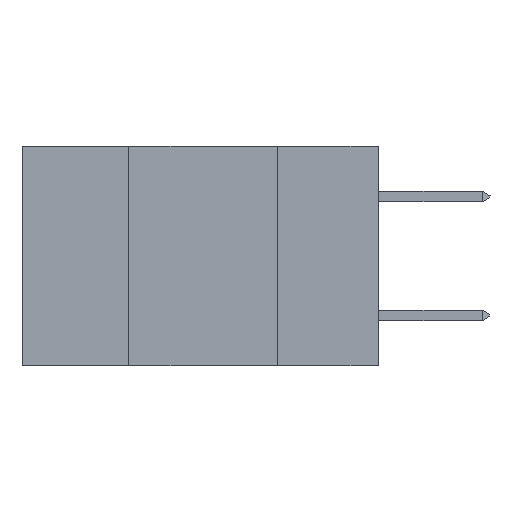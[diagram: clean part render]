
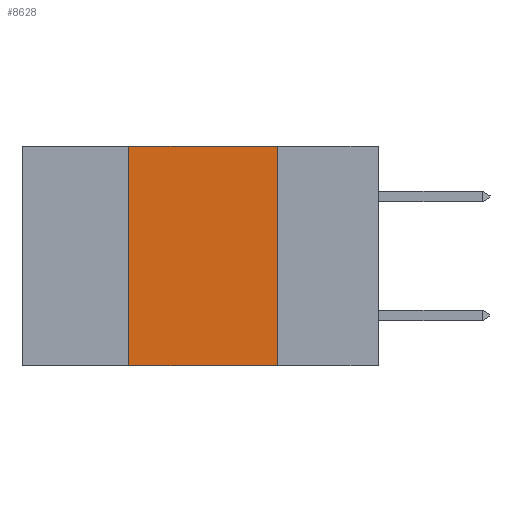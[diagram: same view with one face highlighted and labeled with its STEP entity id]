
A CAD part, left-side view. The second image highlights one B-rep face of the part: STEP entity #8628.
In plain terms, the highlighted planar face has unit normal (-1, 0, 0).
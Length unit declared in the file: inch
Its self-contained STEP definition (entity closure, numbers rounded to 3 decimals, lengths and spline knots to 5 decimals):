
#467 = CARTESIAN_POINT ( 'NONE',  ( 0., 0.6, 0. ) ) ;
#910 = CARTESIAN_POINT ( 'NONE',  ( 0., 0.17, -0.37 ) ) ;
#999 = ORIENTED_EDGE ( 'NONE', *, *, #2778, .F. ) ;
#1193 = CARTESIAN_POINT ( 'NONE',  ( 0., 0.17, -0.37 ) ) ;
#1244 = EDGE_CURVE ( 'NONE', #10765, #5327, #7498, .T. ) ;
#1844 = LINE ( 'NONE', #2875, #10966 ) ;
#1901 = ORIENTED_EDGE ( 'NONE', *, *, #1244, .T. ) ;
#2778 = EDGE_CURVE ( 'NONE', #9141, #6094, #1844, .T. ) ;
#2875 = CARTESIAN_POINT ( 'NONE',  ( 0., 0.6, 0. ) ) ;
#2904 = LINE ( 'NONE', #9290, #5956 ) ;
#3228 = VECTOR ( 'NONE', #5620, 39.37008 ) ;
#3289 = VECTOR ( 'NONE', #4415, 39.37008 ) ;
#4415 = DIRECTION ( 'NONE',  ( 0., -1., 0. ) ) ;
#4650 = CARTESIAN_POINT ( 'NONE',  ( 0., 0.42, 0. ) ) ;
#4996 = ORIENTED_EDGE ( 'NONE', *, *, #7415, .F. ) ;
#5112 = DIRECTION ( 'NONE',  ( 0., 0., 1. ) ) ;
#5327 = VERTEX_POINT ( 'NONE', #910 ) ;
#5620 = DIRECTION ( 'NONE',  ( 0., 0., -1. ) ) ;
#5935 = DIRECTION ( 'NONE',  ( 0., 0., -1. ) ) ;
#5956 = VECTOR ( 'NONE', #5112, 39.37008 ) ;
#5997 = FACE_OUTER_BOUND ( 'NONE', #9221, .T. ) ;
#6094 = VERTEX_POINT ( 'NONE', #6253 ) ;
#6253 = CARTESIAN_POINT ( 'NONE',  ( 0., 0.17, 0. ) ) ;
#6644 = LINE ( 'NONE', #1193, #3228 ) ;
#7415 = EDGE_CURVE ( 'NONE', #6094, #5327, #6644, .T. ) ;
#7498 = LINE ( 'NONE', #8006, #3289 ) ;
#8006 = CARTESIAN_POINT ( 'NONE',  ( 0., 0.6, -0.37 ) ) ;
#8025 = CARTESIAN_POINT ( 'NONE',  ( 0., 0.42, -0.37 ) ) ;
#8346 = DIRECTION ( 'NONE',  ( 0., -1., 0. ) ) ;
#8628 = ADVANCED_FACE ( 'NONE', ( #5997 ), #8704, .F. ) ;
#8704 = PLANE ( 'NONE',  #10124 ) ;
#8837 = EDGE_CURVE ( 'NONE', #10765, #9141, #2904, .T. ) ;
#9141 = VERTEX_POINT ( 'NONE', #4650 ) ;
#9221 = EDGE_LOOP ( 'NONE', ( #4996, #999, #9645, #1901 ) ) ;
#9290 = CARTESIAN_POINT ( 'NONE',  ( 0., 0.42, -0.37 ) ) ;
#9645 = ORIENTED_EDGE ( 'NONE', *, *, #8837, .F. ) ;
#10124 = AXIS2_PLACEMENT_3D ( 'NONE', #467, #11459, #5935 ) ;
#10765 = VERTEX_POINT ( 'NONE', #8025 ) ;
#10966 = VECTOR ( 'NONE', #8346, 39.37008 ) ;
#11459 = DIRECTION ( 'NONE',  ( 1., 0., 0. ) ) ;
